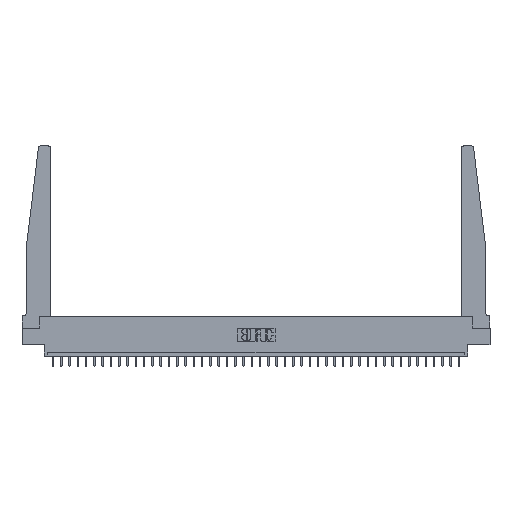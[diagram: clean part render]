
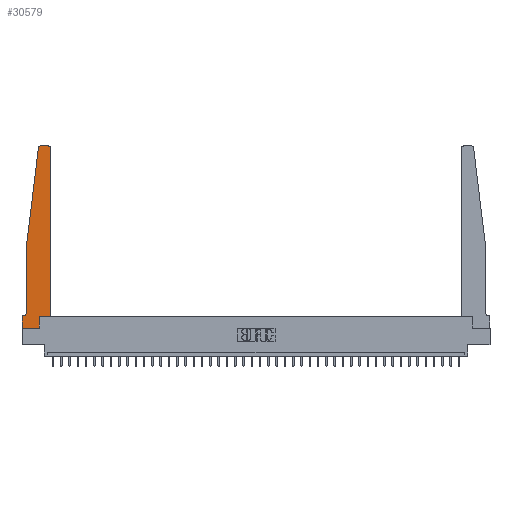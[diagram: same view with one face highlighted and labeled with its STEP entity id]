
A CAD part, top view. The second image highlights one B-rep face of the part: STEP entity #30579.
In plain terms, the highlighted planar face has unit normal (0, 0, 1).
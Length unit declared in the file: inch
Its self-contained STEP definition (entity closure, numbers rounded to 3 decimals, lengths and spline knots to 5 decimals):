
#200 = PLANE ( 'NONE',  #15157 ) ;
#305 = ORIENTED_EDGE ( 'NONE', *, *, #2737, .T. ) ;
#1072 = DIRECTION ( 'NONE',  ( -0.122, -0.992, 0. ) ) ;
#1691 = DIRECTION ( 'NONE',  ( -1., 0., 0. ) ) ;
#2644 = CARTESIAN_POINT ( 'NONE',  ( 0., 0., 0.37 ) ) ;
#2737 = EDGE_CURVE ( 'NONE', #33558, #27056, #10506, .T. ) ;
#2794 = VERTEX_POINT ( 'NONE', #16768 ) ;
#3323 = LINE ( 'NONE', #20312, #4052 ) ;
#3328 = CARTESIAN_POINT ( 'NONE',  ( 0., 0., 0.37 ) ) ;
#3456 = EDGE_CURVE ( 'NONE', #4403, #33112, #34355, .T. ) ;
#3506 = LINE ( 'NONE', #3328, #4805 ) ;
#3697 = EDGE_CURVE ( 'NONE', #4997, #30136, #3758, .T. ) ;
#3758 = LINE ( 'NONE', #14669, #11130 ) ;
#3833 = EDGE_CURVE ( 'NONE', #34059, #33558, #6960, .T. ) ;
#4052 = VECTOR ( 'NONE', #19788, 39.37008 ) ;
#4317 = CARTESIAN_POINT ( 'NONE',  ( 0.015, 0.2375, 0.37 ) ) ;
#4403 = VERTEX_POINT ( 'NONE', #11529 ) ;
#4536 = CARTESIAN_POINT ( 'NONE',  ( 0.065, 0.1875, 0.37 ) ) ;
#4805 = VECTOR ( 'NONE', #19616, 39.37008 ) ;
#4883 = DIRECTION ( 'NONE',  ( 1., 0., 0. ) ) ;
#4997 = VERTEX_POINT ( 'NONE', #7010 ) ;
#5171 = CARTESIAN_POINT ( 'NONE',  ( 0.2605, 0.18, 0.37 ) ) ;
#5231 = DIRECTION ( 'NONE',  ( 0., 0., 1. ) ) ;
#5384 = ORIENTED_EDGE ( 'NONE', *, *, #11934, .T. ) ;
#5463 = DIRECTION ( 'NONE',  ( 1., 0., 0. ) ) ;
#5817 = EDGE_CURVE ( 'NONE', #2794, #22439, #7232, .T. ) ;
#6377 = EDGE_CURVE ( 'NONE', #30136, #18619, #3323, .T. ) ;
#6960 = LINE ( 'NONE', #10327, #24878 ) ;
#7010 = CARTESIAN_POINT ( 'NONE',  ( 0.24675, 2.72367, 0.37 ) ) ;
#7192 = ORIENTED_EDGE ( 'NONE', *, *, #6377, .T. ) ;
#7232 = LINE ( 'NONE', #4536, #11680 ) ;
#7559 = CARTESIAN_POINT ( 'NONE',  ( 0.27653, 2.75, 0.37 ) ) ;
#7668 = VECTOR ( 'NONE', #9901, 39.37008 ) ;
#8001 = CARTESIAN_POINT ( 'NONE',  ( 0.065, 0.2375, 0.37 ) ) ;
#9901 = DIRECTION ( 'NONE',  ( -1., 0., 0. ) ) ;
#10035 = VECTOR ( 'NONE', #15911, 39.37008 ) ;
#10327 = CARTESIAN_POINT ( 'NONE',  ( 0.2605, 0.18, 0.37 ) ) ;
#10414 = CARTESIAN_POINT ( 'NONE',  ( 0.27653, 2.72, 0.37 ) ) ;
#10499 = EDGE_LOOP ( 'NONE', ( #32533, #11103, #26698, #7192, #5384, #27737, #26786, #22106, #20044, #305, #22939, #17018 ) ) ;
#10506 = LINE ( 'NONE', #32298, #12186 ) ;
#10767 = CARTESIAN_POINT ( 'NONE',  ( 0.2605, 0., 0.37 ) ) ;
#10891 = CIRCLE ( 'NONE', #11452, 0.03 ) ;
#11085 = CARTESIAN_POINT ( 'NONE',  ( 0.425, 0.18, 0.37 ) ) ;
#11098 = DIRECTION ( 'NONE',  ( 0., 0., 1. ) ) ;
#11103 = ORIENTED_EDGE ( 'NONE', *, *, #25179, .T. ) ;
#11130 = VECTOR ( 'NONE', #1072, 39.37008 ) ;
#11452 = AXIS2_PLACEMENT_3D ( 'NONE', #10414, #5231, #4883 ) ;
#11527 = DIRECTION ( 'NONE',  ( 0., 0., 1. ) ) ;
#11529 = CARTESIAN_POINT ( 'NONE',  ( 0.395, 2.75, 0.37 ) ) ;
#11680 = VECTOR ( 'NONE', #1691, 39.37008 ) ;
#11934 = EDGE_CURVE ( 'NONE', #18619, #2794, #32797, .T. ) ;
#12186 = VECTOR ( 'NONE', #21425, 39.37008 ) ;
#12862 = EDGE_CURVE ( 'NONE', #34949, #4403, #18559, .T. ) ;
#12976 = VECTOR ( 'NONE', #21962, 39.37008 ) ;
#13201 = EDGE_CURVE ( 'NONE', #27056, #34949, #29672, .T. ) ;
#13492 = VERTEX_POINT ( 'NONE', #18209 ) ;
#13979 = FACE_OUTER_BOUND ( 'NONE', #10499, .T. ) ;
#14188 = CARTESIAN_POINT ( 'NONE',  ( 0.065, 1.25, 0.37 ) ) ;
#14669 = CARTESIAN_POINT ( 'NONE',  ( 0.065, 1.25, 0.37 ) ) ;
#14871 = DIRECTION ( 'NONE',  ( -1., 0., 0. ) ) ;
#15157 = AXIS2_PLACEMENT_3D ( 'NONE', #27202, #11098, #24886 ) ;
#15911 = DIRECTION ( 'NONE',  ( 0., 1., 0. ) ) ;
#16365 = CARTESIAN_POINT ( 'NONE',  ( 0.395, 2.72, 0.37 ) ) ;
#16583 = CARTESIAN_POINT ( 'NONE',  ( 0.425, 2.72, 0.37 ) ) ;
#16768 = CARTESIAN_POINT ( 'NONE',  ( 0.015, 0.1875, 0.37 ) ) ;
#17018 = ORIENTED_EDGE ( 'NONE', *, *, #12862, .T. ) ;
#17486 = EDGE_CURVE ( 'NONE', #13492, #34059, #19099, .T. ) ;
#18209 = CARTESIAN_POINT ( 'NONE',  ( 0., 0., 0.37 ) ) ;
#18559 = CIRCLE ( 'NONE', #33940, 0.03 ) ;
#18619 = VERTEX_POINT ( 'NONE', #8001 ) ;
#19099 = LINE ( 'NONE', #2644, #12976 ) ;
#19616 = DIRECTION ( 'NONE',  ( 0., -1., 0. ) ) ;
#19788 = DIRECTION ( 'NONE',  ( 0., -1., 0. ) ) ;
#20044 = ORIENTED_EDGE ( 'NONE', *, *, #3833, .T. ) ;
#20312 = CARTESIAN_POINT ( 'NONE',  ( 0.065, 1.25, 0.37 ) ) ;
#20833 = AXIS2_PLACEMENT_3D ( 'NONE', #4317, #31635, #14871 ) ;
#21425 = DIRECTION ( 'NONE',  ( 1., 0., 0. ) ) ;
#21962 = DIRECTION ( 'NONE',  ( 1., 0., 0. ) ) ;
#22106 = ORIENTED_EDGE ( 'NONE', *, *, #17486, .T. ) ;
#22439 = VERTEX_POINT ( 'NONE', #22574 ) ;
#22574 = CARTESIAN_POINT ( 'NONE',  ( 0., 0.1875, 0.37 ) ) ;
#22939 = ORIENTED_EDGE ( 'NONE', *, *, #13201, .T. ) ;
#24878 = VECTOR ( 'NONE', #32122, 39.37008 ) ;
#24886 = DIRECTION ( 'NONE',  ( 1., 0., 0. ) ) ;
#25179 = EDGE_CURVE ( 'NONE', #33112, #4997, #10891, .T. ) ;
#26698 = ORIENTED_EDGE ( 'NONE', *, *, #3697, .T. ) ;
#26786 = ORIENTED_EDGE ( 'NONE', *, *, #30939, .T. ) ;
#27056 = VERTEX_POINT ( 'NONE', #31658 ) ;
#27202 = CARTESIAN_POINT ( 'NONE',  ( 0., 0.1875, 0.37 ) ) ;
#27737 = ORIENTED_EDGE ( 'NONE', *, *, #5817, .T. ) ;
#29672 = LINE ( 'NONE', #11085, #10035 ) ;
#30136 = VERTEX_POINT ( 'NONE', #14188 ) ;
#30579 = ADVANCED_FACE ( 'NONE', ( #13979 ), #200, .T. ) ;
#30939 = EDGE_CURVE ( 'NONE', #22439, #13492, #3506, .T. ) ;
#31000 = CARTESIAN_POINT ( 'NONE',  ( 0.25, 2.75, 0.37 ) ) ;
#31635 = DIRECTION ( 'NONE',  ( 0., 0., -1. ) ) ;
#31658 = CARTESIAN_POINT ( 'NONE',  ( 0.425, 0.18, 0.37 ) ) ;
#32122 = DIRECTION ( 'NONE',  ( 0., 1., 0. ) ) ;
#32298 = CARTESIAN_POINT ( 'NONE',  ( 0.425, 0.18, 0.37 ) ) ;
#32533 = ORIENTED_EDGE ( 'NONE', *, *, #3456, .T. ) ;
#32797 = CIRCLE ( 'NONE', #20833, 0.05 ) ;
#33112 = VERTEX_POINT ( 'NONE', #7559 ) ;
#33558 = VERTEX_POINT ( 'NONE', #5171 ) ;
#33940 = AXIS2_PLACEMENT_3D ( 'NONE', #16365, #11527, #5463 ) ;
#34059 = VERTEX_POINT ( 'NONE', #10767 ) ;
#34355 = LINE ( 'NONE', #31000, #7668 ) ;
#34949 = VERTEX_POINT ( 'NONE', #16583 ) ;
